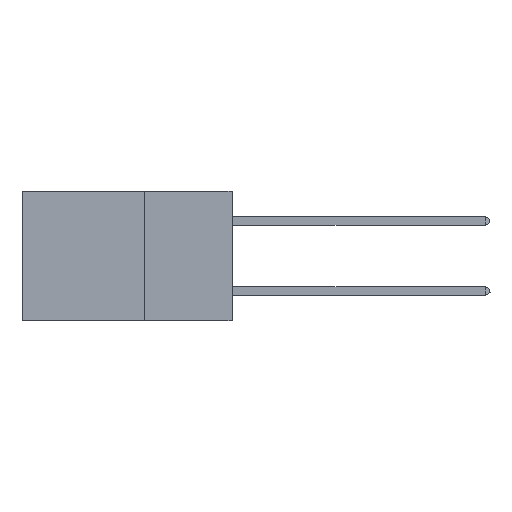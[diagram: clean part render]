
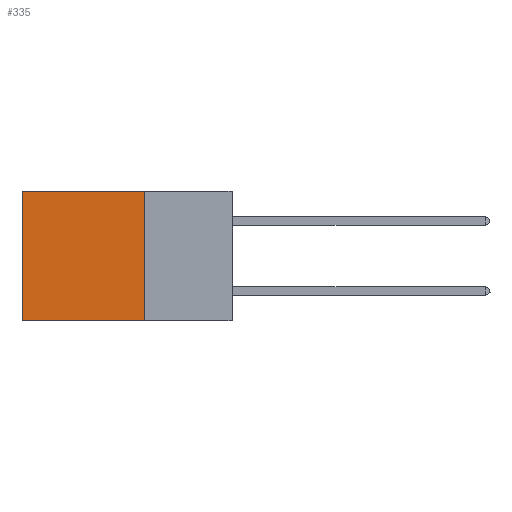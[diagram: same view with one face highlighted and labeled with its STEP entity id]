
A CAD part, left-side view. The second image highlights one B-rep face of the part: STEP entity #335.
In plain terms, the highlighted planar face has unit normal (-1, 0, 0).
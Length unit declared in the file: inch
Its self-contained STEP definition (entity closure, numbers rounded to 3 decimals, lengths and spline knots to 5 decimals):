
#335 = ADVANCED_FACE ( 'NONE', ( #2655 ), #23052, .F. ) ;
#731 = VECTOR ( 'NONE', #11731, 39.37008 ) ;
#1165 = CARTESIAN_POINT ( 'NONE',  ( 0.2875, 0.6, 0. ) ) ;
#1347 = EDGE_LOOP ( 'NONE', ( #26153, #24987, #28264, #11780 ) ) ;
#2655 = FACE_OUTER_BOUND ( 'NONE', #1347, .T. ) ;
#4205 = EDGE_CURVE ( 'NONE', #21902, #14572, #21645, .T. ) ;
#7024 = LINE ( 'NONE', #29051, #27190 ) ;
#9263 = CARTESIAN_POINT ( 'NONE',  ( 0.2875, 0.25, -0.37 ) ) ;
#9977 = DIRECTION ( 'NONE',  ( 0., 1., 0. ) ) ;
#10915 = DIRECTION ( 'NONE',  ( 1., 0., 0. ) ) ;
#11731 = DIRECTION ( 'NONE',  ( 0., 0., -1. ) ) ;
#11780 = ORIENTED_EDGE ( 'NONE', *, *, #14739, .T. ) ;
#11859 = LINE ( 'NONE', #30411, #18405 ) ;
#14572 = VERTEX_POINT ( 'NONE', #9263 ) ;
#14739 = EDGE_CURVE ( 'NONE', #21902, #28805, #11859, .T. ) ;
#16082 = CARTESIAN_POINT ( 'NONE',  ( 0.2875, 0.25, 0. ) ) ;
#18147 = DIRECTION ( 'NONE',  ( 0., 0., -1. ) ) ;
#18405 = VECTOR ( 'NONE', #30299, 39.37008 ) ;
#18563 = EDGE_CURVE ( 'NONE', #14572, #25574, #7024, .T. ) ;
#18785 = CARTESIAN_POINT ( 'NONE',  ( 0.2875, 0.25, 0. ) ) ;
#19186 = CARTESIAN_POINT ( 'NONE',  ( 0.2875, 0.25, 0. ) ) ;
#20403 = CARTESIAN_POINT ( 'NONE',  ( 0.2875, 0.6, 0. ) ) ;
#21645 = LINE ( 'NONE', #19186, #731 ) ;
#21902 = VERTEX_POINT ( 'NONE', #18785 ) ;
#22398 = CARTESIAN_POINT ( 'NONE',  ( 0.2875, 0.6, -0.37 ) ) ;
#23049 = LINE ( 'NONE', #1165, #24970 ) ;
#23052 = PLANE ( 'NONE',  #28730 ) ;
#24970 = VECTOR ( 'NONE', #25984, 39.37008 ) ;
#24987 = ORIENTED_EDGE ( 'NONE', *, *, #18563, .F. ) ;
#25574 = VERTEX_POINT ( 'NONE', #22398 ) ;
#25984 = DIRECTION ( 'NONE',  ( 0., 0., -1. ) ) ;
#26153 = ORIENTED_EDGE ( 'NONE', *, *, #27103, .T. ) ;
#27103 = EDGE_CURVE ( 'NONE', #28805, #25574, #23049, .T. ) ;
#27190 = VECTOR ( 'NONE', #9977, 39.37008 ) ;
#28264 = ORIENTED_EDGE ( 'NONE', *, *, #4205, .F. ) ;
#28730 = AXIS2_PLACEMENT_3D ( 'NONE', #16082, #10915, #18147 ) ;
#28805 = VERTEX_POINT ( 'NONE', #20403 ) ;
#29051 = CARTESIAN_POINT ( 'NONE',  ( 0.2875, 0.25, -0.37 ) ) ;
#30299 = DIRECTION ( 'NONE',  ( 0., 1., 0. ) ) ;
#30411 = CARTESIAN_POINT ( 'NONE',  ( 0.2875, 0.25, 0. ) ) ;
